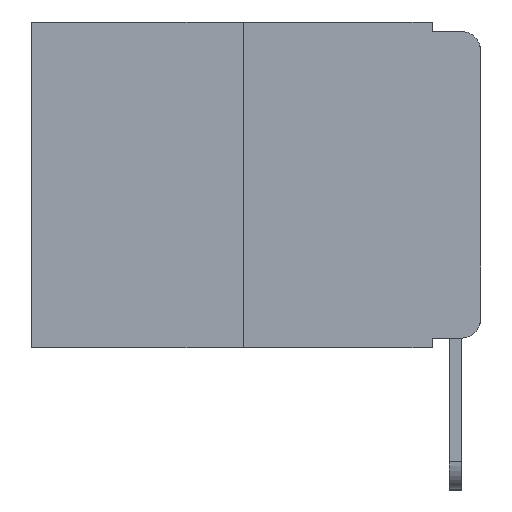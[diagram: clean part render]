
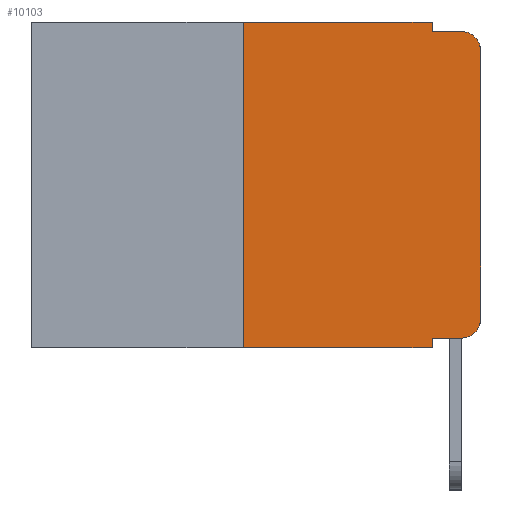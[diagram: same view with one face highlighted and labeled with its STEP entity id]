
A CAD part, left-side view. The second image highlights one B-rep face of the part: STEP entity #10103.
In plain terms, the highlighted planar face has unit normal (-1, 0, 0).
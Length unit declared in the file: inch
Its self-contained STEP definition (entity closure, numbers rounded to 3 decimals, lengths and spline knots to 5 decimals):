
#26 = DIRECTION ( 'NONE',  ( 0., -1., 0. ) ) ;
#62 = DIRECTION ( 'NONE',  ( 0., 0., 1. ) ) ;
#236 = EDGE_LOOP ( 'NONE', ( #7690, #2835, #1341, #5469, #1751, #1919, #10051, #6602, #8411, #6125 ) ) ;
#244 = EDGE_CURVE ( 'NONE', #2437, #5442, #1618, .T. ) ;
#285 = AXIS2_PLACEMENT_3D ( 'NONE', #1198, #7721, #514 ) ;
#514 = DIRECTION ( 'NONE',  ( 0., 0., -1. ) ) ;
#605 = VECTOR ( 'NONE', #26, 39.37008 ) ;
#619 = DIRECTION ( 'NONE',  ( -1., 0., 0. ) ) ;
#723 = EDGE_CURVE ( 'NONE', #1595, #3487, #1900, .T. ) ;
#819 = EDGE_CURVE ( 'NONE', #1595, #5442, #4078, .T. ) ;
#833 = CARTESIAN_POINT ( 'NONE',  ( 0., 0.051, -0.333 ) ) ;
#963 = CARTESIAN_POINT ( 'NONE',  ( 0., 0.25, -0.343 ) ) ;
#978 = CARTESIAN_POINT ( 'NONE',  ( 0., 0.051, -0.343 ) ) ;
#1148 = DIRECTION ( 'NONE',  ( 0., -1., 0. ) ) ;
#1198 = CARTESIAN_POINT ( 'NONE',  ( 0., 0.473, 0. ) ) ;
#1248 = LINE ( 'NONE', #3790, #4152 ) ;
#1341 = ORIENTED_EDGE ( 'NONE', *, *, #6240, .F. ) ;
#1594 = CARTESIAN_POINT ( 'NONE',  ( 0., 0., 0. ) ) ;
#1595 = VERTEX_POINT ( 'NONE', #963 ) ;
#1618 = LINE ( 'NONE', #4857, #4383 ) ;
#1624 = CARTESIAN_POINT ( 'NONE',  ( 0., 0.051, -0.01 ) ) ;
#1634 = AXIS2_PLACEMENT_3D ( 'NONE', #6208, #3700, #4492 ) ;
#1694 = LINE ( 'NONE', #5178, #10379 ) ;
#1751 = ORIENTED_EDGE ( 'NONE', *, *, #5091, .F. ) ;
#1900 = LINE ( 'NONE', #9791, #9663 ) ;
#1919 = ORIENTED_EDGE ( 'NONE', *, *, #723, .F. ) ;
#2077 = CARTESIAN_POINT ( 'NONE',  ( 0., 0.25, 0. ) ) ;
#2173 = FACE_OUTER_BOUND ( 'NONE', #236, .T. ) ;
#2260 = DIRECTION ( 'NONE',  ( 0., 0., -1. ) ) ;
#2379 = CARTESIAN_POINT ( 'NONE',  ( 0., 0.02, -0.03 ) ) ;
#2437 = VERTEX_POINT ( 'NONE', #9025 ) ;
#2835 = ORIENTED_EDGE ( 'NONE', *, *, #8939, .T. ) ;
#2847 = AXIS2_PLACEMENT_3D ( 'NONE', #2379, #619, #4059 ) ;
#3277 = CARTESIAN_POINT ( 'NONE',  ( 0., 0.473, -0.343 ) ) ;
#3373 = LINE ( 'NONE', #5155, #3844 ) ;
#3487 = VERTEX_POINT ( 'NONE', #2077 ) ;
#3700 = DIRECTION ( 'NONE',  ( -1., 0., 0. ) ) ;
#3790 = CARTESIAN_POINT ( 'NONE',  ( 0., 0.473, 0. ) ) ;
#3844 = VECTOR ( 'NONE', #4381, 39.37008 ) ;
#4059 = DIRECTION ( 'NONE',  ( 0., 0., -1. ) ) ;
#4078 = LINE ( 'NONE', #3277, #605 ) ;
#4103 = CARTESIAN_POINT ( 'NONE',  ( 0., 0., -0.313 ) ) ;
#4152 = VECTOR ( 'NONE', #1148, 39.37008 ) ;
#4381 = DIRECTION ( 'NONE',  ( 0., -1., 0. ) ) ;
#4383 = VECTOR ( 'NONE', #2260, 39.37008 ) ;
#4421 = CARTESIAN_POINT ( 'NONE',  ( 0., 0.02, -0.01 ) ) ;
#4492 = DIRECTION ( 'NONE',  ( 0., 0., -1. ) ) ;
#4638 = CARTESIAN_POINT ( 'NONE',  ( 0., 0.051, 0. ) ) ;
#4857 = CARTESIAN_POINT ( 'NONE',  ( 0., 0.051, 0. ) ) ;
#4898 = DIRECTION ( 'NONE',  ( 0., 0., 1. ) ) ;
#5027 = DIRECTION ( 'NONE',  ( 0., 0., -1. ) ) ;
#5091 = EDGE_CURVE ( 'NONE', #3487, #9244, #1248, .T. ) ;
#5155 = CARTESIAN_POINT ( 'NONE',  ( 0., 0.051, -0.01 ) ) ;
#5178 = CARTESIAN_POINT ( 'NONE',  ( 0., 0.051, 0. ) ) ;
#5411 = PLANE ( 'NONE',  #285 ) ;
#5442 = VERTEX_POINT ( 'NONE', #978 ) ;
#5469 = ORIENTED_EDGE ( 'NONE', *, *, #9160, .F. ) ;
#5883 = CARTESIAN_POINT ( 'NONE',  ( 0., 0.02, -0.333 ) ) ;
#6125 = ORIENTED_EDGE ( 'NONE', *, *, #8385, .T. ) ;
#6208 = CARTESIAN_POINT ( 'NONE',  ( 0., 0.02, -0.313 ) ) ;
#6240 = EDGE_CURVE ( 'NONE', #9465, #10361, #3373, .T. ) ;
#6278 = VERTEX_POINT ( 'NONE', #5883 ) ;
#6602 = ORIENTED_EDGE ( 'NONE', *, *, #244, .F. ) ;
#7630 = VECTOR ( 'NONE', #9607, 39.37008 ) ;
#7690 = ORIENTED_EDGE ( 'NONE', *, *, #8483, .T. ) ;
#7721 = DIRECTION ( 'NONE',  ( 1., 0., 0. ) ) ;
#8285 = CIRCLE ( 'NONE', #1634, 0.02 ) ;
#8291 = VECTOR ( 'NONE', #62, 39.37008 ) ;
#8385 = EDGE_CURVE ( 'NONE', #6278, #8985, #8285, .T. ) ;
#8411 = ORIENTED_EDGE ( 'NONE', *, *, #10179, .T. ) ;
#8483 = EDGE_CURVE ( 'NONE', #8985, #8780, #10539, .T. ) ;
#8780 = VERTEX_POINT ( 'NONE', #10094 ) ;
#8939 = EDGE_CURVE ( 'NONE', #8780, #10361, #9143, .T. ) ;
#8985 = VERTEX_POINT ( 'NONE', #4103 ) ;
#9025 = CARTESIAN_POINT ( 'NONE',  ( 0., 0.051, -0.333 ) ) ;
#9143 = CIRCLE ( 'NONE', #2847, 0.02 ) ;
#9160 = EDGE_CURVE ( 'NONE', #9244, #9465, #1694, .T. ) ;
#9244 = VERTEX_POINT ( 'NONE', #4638 ) ;
#9465 = VERTEX_POINT ( 'NONE', #1624 ) ;
#9607 = DIRECTION ( 'NONE',  ( 0., -1., 0. ) ) ;
#9663 = VECTOR ( 'NONE', #4898, 39.37008 ) ;
#9791 = CARTESIAN_POINT ( 'NONE',  ( 0., 0.25, 0. ) ) ;
#10051 = ORIENTED_EDGE ( 'NONE', *, *, #819, .T. ) ;
#10094 = CARTESIAN_POINT ( 'NONE',  ( 0., 0., -0.03 ) ) ;
#10103 = ADVANCED_FACE ( 'NONE', ( #2173 ), #5411, .F. ) ;
#10179 = EDGE_CURVE ( 'NONE', #2437, #6278, #10525, .T. ) ;
#10361 = VERTEX_POINT ( 'NONE', #4421 ) ;
#10379 = VECTOR ( 'NONE', #5027, 39.37008 ) ;
#10525 = LINE ( 'NONE', #833, #7630 ) ;
#10539 = LINE ( 'NONE', #1594, #8291 ) ;
